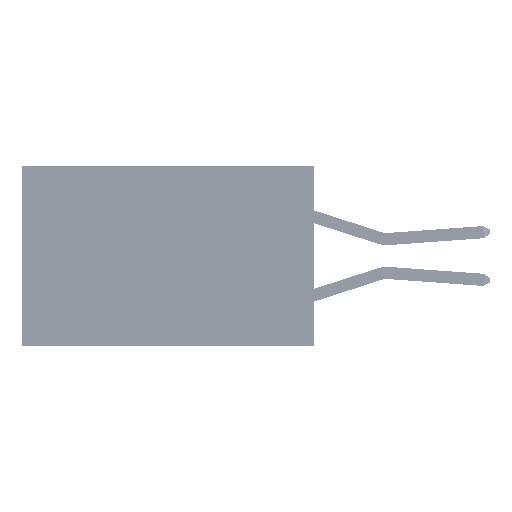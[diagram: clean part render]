
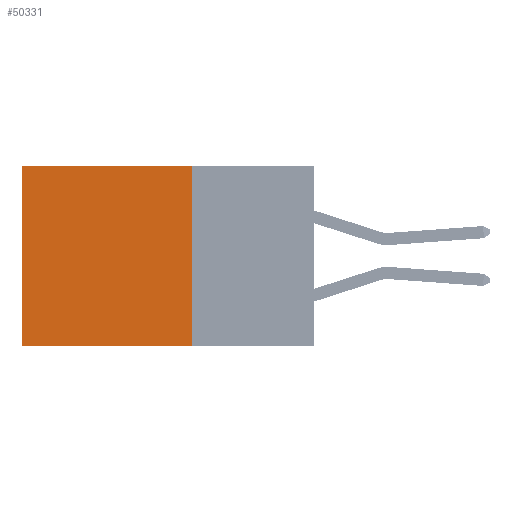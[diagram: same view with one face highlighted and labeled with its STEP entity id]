
A CAD part, left-side view. The second image highlights one B-rep face of the part: STEP entity #50331.
In plain terms, the highlighted planar face has unit normal (-1, 0, 0).
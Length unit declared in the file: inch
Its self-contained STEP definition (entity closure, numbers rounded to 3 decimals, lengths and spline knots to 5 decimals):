
#480 = VERTEX_POINT ( 'NONE', #15888 ) ;
#1012 = CARTESIAN_POINT ( 'NONE',  ( 0.2875, 0.25, -0.37 ) ) ;
#2648 = VECTOR ( 'NONE', #40658, 39.37008 ) ;
#3368 = LINE ( 'NONE', #28008, #48404 ) ;
#3811 = LINE ( 'NONE', #16006, #2648 ) ;
#3864 = VERTEX_POINT ( 'NONE', #27162 ) ;
#3877 = DIRECTION ( 'NONE',  ( 0., 0., -1. ) ) ;
#7006 = VECTOR ( 'NONE', #44321, 39.37008 ) ;
#8420 = FACE_OUTER_BOUND ( 'NONE', #20498, .T. ) ;
#13838 = CARTESIAN_POINT ( 'NONE',  ( 0.2875, 0.25, 0. ) ) ;
#14926 = ORIENTED_EDGE ( 'NONE', *, *, #44579, .T. ) ;
#15888 = CARTESIAN_POINT ( 'NONE',  ( 0.2875, 0.6, 0. ) ) ;
#15959 = LINE ( 'NONE', #48293, #7006 ) ;
#16006 = CARTESIAN_POINT ( 'NONE',  ( 0.2875, 0.25, -0.37 ) ) ;
#16570 = ORIENTED_EDGE ( 'NONE', *, *, #18256, .T. ) ;
#16621 = PLANE ( 'NONE',  #20579 ) ;
#16901 = EDGE_CURVE ( 'NONE', #48587, #3864, #3811, .T. ) ;
#17274 = DIRECTION ( 'NONE',  ( 0., 1., 0. ) ) ;
#18256 = EDGE_CURVE ( 'NONE', #480, #3864, #3368, .T. ) ;
#20498 = EDGE_LOOP ( 'NONE', ( #16570, #24396, #26647, #14926 ) ) ;
#20579 = AXIS2_PLACEMENT_3D ( 'NONE', #41522, #21652, #33555 ) ;
#21525 = LINE ( 'NONE', #13838, #27890 ) ;
#21652 = DIRECTION ( 'NONE',  ( 1., 0., 0. ) ) ;
#24396 = ORIENTED_EDGE ( 'NONE', *, *, #16901, .F. ) ;
#26647 = ORIENTED_EDGE ( 'NONE', *, *, #49391, .F. ) ;
#27162 = CARTESIAN_POINT ( 'NONE',  ( 0.2875, 0.6, -0.37 ) ) ;
#27890 = VECTOR ( 'NONE', #17274, 39.37008 ) ;
#28008 = CARTESIAN_POINT ( 'NONE',  ( 0.2875, 0.6, 0. ) ) ;
#33555 = DIRECTION ( 'NONE',  ( 0., 0., -1. ) ) ;
#40658 = DIRECTION ( 'NONE',  ( 0., 1., 0. ) ) ;
#41522 = CARTESIAN_POINT ( 'NONE',  ( 0.2875, 0.25, 0. ) ) ;
#44321 = DIRECTION ( 'NONE',  ( 0., 0., -1. ) ) ;
#44579 = EDGE_CURVE ( 'NONE', #47172, #480, #21525, .T. ) ;
#47172 = VERTEX_POINT ( 'NONE', #51836 ) ;
#48293 = CARTESIAN_POINT ( 'NONE',  ( 0.2875, 0.25, 0. ) ) ;
#48404 = VECTOR ( 'NONE', #3877, 39.37008 ) ;
#48587 = VERTEX_POINT ( 'NONE', #1012 ) ;
#49391 = EDGE_CURVE ( 'NONE', #47172, #48587, #15959, .T. ) ;
#50331 = ADVANCED_FACE ( 'NONE', ( #8420 ), #16621, .F. ) ;
#51836 = CARTESIAN_POINT ( 'NONE',  ( 0.2875, 0.25, 0. ) ) ;
